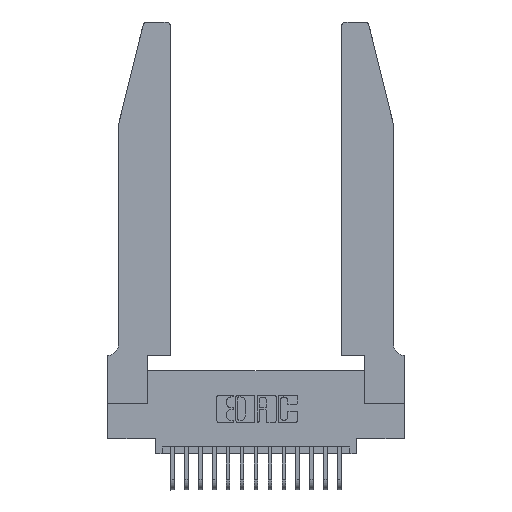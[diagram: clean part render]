
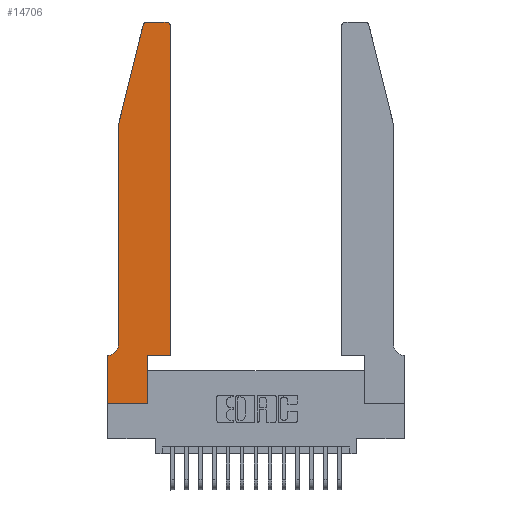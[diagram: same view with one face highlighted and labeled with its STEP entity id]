
A CAD part, top view. The second image highlights one B-rep face of the part: STEP entity #14706.
In plain terms, the highlighted planar face has unit normal (0, 0, 1).
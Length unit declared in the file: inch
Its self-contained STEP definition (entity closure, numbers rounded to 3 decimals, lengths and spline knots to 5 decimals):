
#154 = CIRCLE ( 'NONE', #2143, 0.03 ) ;
#190 = CARTESIAN_POINT ( 'NONE',  ( 0., 0.35, 0.37 ) ) ;
#294 = ORIENTED_EDGE ( 'NONE', *, *, #7424, .T. ) ;
#326 = CARTESIAN_POINT ( 'NONE',  ( 0.0755, 0.42, 0.37 ) ) ;
#828 = LINE ( 'NONE', #13875, #15801 ) ;
#1557 = VERTEX_POINT ( 'NONE', #5590 ) ;
#1702 = ORIENTED_EDGE ( 'NONE', *, *, #6084, .T. ) ;
#1766 = DIRECTION ( 'NONE',  ( 1., 0., 0. ) ) ;
#1769 = LINE ( 'NONE', #11265, #7815 ) ;
#1826 = CARTESIAN_POINT ( 'NONE',  ( 0.2865, 0.35, 0.37 ) ) ;
#1850 = VERTEX_POINT ( 'NONE', #4550 ) ;
#2143 = AXIS2_PLACEMENT_3D ( 'NONE', #6010, #15923, #7480 ) ;
#2507 = FACE_OUTER_BOUND ( 'NONE', #15853, .T. ) ;
#2542 = EDGE_CURVE ( 'NONE', #5289, #15645, #154, .T. ) ;
#2556 = ORIENTED_EDGE ( 'NONE', *, *, #13626, .T. ) ;
#2882 = AXIS2_PLACEMENT_3D ( 'NONE', #8494, #18285, #9923 ) ;
#2989 = LINE ( 'NONE', #3515, #9884 ) ;
#3036 = VERTEX_POINT ( 'NONE', #9968 ) ;
#3207 = PLANE ( 'NONE',  #17523 ) ;
#3515 = CARTESIAN_POINT ( 'NONE',  ( 0.4505, 0.35, 0.37 ) ) ;
#3634 = VERTEX_POINT ( 'NONE', #12335 ) ;
#3712 = EDGE_CURVE ( 'NONE', #3036, #1557, #828, .T. ) ;
#3813 = DIRECTION ( 'NONE',  ( 0., -1., 0. ) ) ;
#4016 = ORIENTED_EDGE ( 'NONE', *, *, #12811, .T. ) ;
#4052 = LINE ( 'NONE', #1826, #17839 ) ;
#4151 = CARTESIAN_POINT ( 'NONE',  ( 0.0055, 0.35, 0.37 ) ) ;
#4157 = ORIENTED_EDGE ( 'NONE', *, *, #9120, .T. ) ;
#4394 = CIRCLE ( 'NONE', #2882, 0.03 ) ;
#4471 = DIRECTION ( 'NONE',  ( -1., 0., 0. ) ) ;
#4533 = CARTESIAN_POINT ( 'NONE',  ( 0.0055, 0.42, 0.37 ) ) ;
#4550 = CARTESIAN_POINT ( 'NONE',  ( 0.4205, 2.75, 0.37 ) ) ;
#5059 = DIRECTION ( 'NONE',  ( 1., 0., 0. ) ) ;
#5289 = VERTEX_POINT ( 'NONE', #13985 ) ;
#5510 = EDGE_CURVE ( 'NONE', #10821, #3036, #15515, .T. ) ;
#5590 = CARTESIAN_POINT ( 'NONE',  ( 0., 0., 0.37 ) ) ;
#5830 = EDGE_CURVE ( 'NONE', #3634, #6228, #6855, .T. ) ;
#5984 = VECTOR ( 'NONE', #13143, 39.37008 ) ;
#6010 = CARTESIAN_POINT ( 'NONE',  ( 0.284, 2.72, 0.37 ) ) ;
#6017 = DIRECTION ( 'NONE',  ( -1., 0., 0. ) ) ;
#6084 = EDGE_CURVE ( 'NONE', #1557, #15093, #17287, .T. ) ;
#6228 = VERTEX_POINT ( 'NONE', #326 ) ;
#6595 = ORIENTED_EDGE ( 'NONE', *, *, #10957, .T. ) ;
#6855 = LINE ( 'NONE', #13909, #14875 ) ;
#7252 = VERTEX_POINT ( 'NONE', #9466 ) ;
#7266 = AXIS2_PLACEMENT_3D ( 'NONE', #4533, #14559, #6017 ) ;
#7424 = EDGE_CURVE ( 'NONE', #16525, #12437, #8203, .T. ) ;
#7480 = DIRECTION ( 'NONE',  ( 1., 0., 0. ) ) ;
#7580 = VECTOR ( 'NONE', #18557, 39.37008 ) ;
#7815 = VECTOR ( 'NONE', #12733, 39.37008 ) ;
#8203 = LINE ( 'NONE', #17210, #15257 ) ;
#8494 = CARTESIAN_POINT ( 'NONE',  ( 0.4205, 2.72, 0.37 ) ) ;
#8720 = CARTESIAN_POINT ( 'NONE',  ( 0.4505, 0.35, 0.37 ) ) ;
#8847 = DIRECTION ( 'NONE',  ( 0., 1., 0. ) ) ;
#9120 = EDGE_CURVE ( 'NONE', #15093, #7252, #4052, .T. ) ;
#9465 = VECTOR ( 'NONE', #4471, 39.37008 ) ;
#9466 = CARTESIAN_POINT ( 'NONE',  ( 0.2865, 0.35, 0.37 ) ) ;
#9628 = CARTESIAN_POINT ( 'NONE',  ( 0.25487, 2.72718, 0.37 ) ) ;
#9884 = VECTOR ( 'NONE', #5059, 39.37008 ) ;
#9907 = LINE ( 'NONE', #14498, #9465 ) ;
#9923 = DIRECTION ( 'NONE',  ( 1., 0., 0. ) ) ;
#9968 = CARTESIAN_POINT ( 'NONE',  ( 0., 0.35, 0.37 ) ) ;
#10329 = ORIENTED_EDGE ( 'NONE', *, *, #3712, .T. ) ;
#10551 = DIRECTION ( 'NONE',  ( 0., 0., 1. ) ) ;
#10821 = VERTEX_POINT ( 'NONE', #4151 ) ;
#10957 = EDGE_CURVE ( 'NONE', #1850, #5289, #9907, .T. ) ;
#11265 = CARTESIAN_POINT ( 'NONE',  ( 0.0755, 2., 0.37 ) ) ;
#11644 = CARTESIAN_POINT ( 'NONE',  ( 0.0755, 0.35, 0.37 ) ) ;
#11752 = CARTESIAN_POINT ( 'NONE',  ( 0., 0., 0.37 ) ) ;
#12335 = CARTESIAN_POINT ( 'NONE',  ( 0.0755, 2., 0.37 ) ) ;
#12437 = VERTEX_POINT ( 'NONE', #16931 ) ;
#12733 = DIRECTION ( 'NONE',  ( -0.239, -0.971, 0. ) ) ;
#12811 = EDGE_CURVE ( 'NONE', #7252, #16525, #2989, .T. ) ;
#13143 = DIRECTION ( 'NONE',  ( 1., 0., 0. ) ) ;
#13166 = CIRCLE ( 'NONE', #7266, 0.07 ) ;
#13374 = ORIENTED_EDGE ( 'NONE', *, *, #17242, .T. ) ;
#13396 = ORIENTED_EDGE ( 'NONE', *, *, #5510, .T. ) ;
#13626 = EDGE_CURVE ( 'NONE', #12437, #1850, #4394, .T. ) ;
#13875 = CARTESIAN_POINT ( 'NONE',  ( 0., 0., 0.37 ) ) ;
#13909 = CARTESIAN_POINT ( 'NONE',  ( 0.0755, 2., 0.37 ) ) ;
#13924 = ORIENTED_EDGE ( 'NONE', *, *, #15940, .T. ) ;
#13985 = CARTESIAN_POINT ( 'NONE',  ( 0.284, 2.75, 0.37 ) ) ;
#14480 = CARTESIAN_POINT ( 'NONE',  ( 0.2865, 0., 0.37 ) ) ;
#14498 = CARTESIAN_POINT ( 'NONE',  ( 0.2605, 2.75, 0.37 ) ) ;
#14559 = DIRECTION ( 'NONE',  ( 0., 0., -1. ) ) ;
#14706 = ADVANCED_FACE ( 'NONE', ( #2507 ), #3207, .T. ) ;
#14875 = VECTOR ( 'NONE', #3813, 39.37008 ) ;
#15093 = VERTEX_POINT ( 'NONE', #14480 ) ;
#15254 = DIRECTION ( 'NONE',  ( 0., -1., 0. ) ) ;
#15257 = VECTOR ( 'NONE', #8847, 39.37008 ) ;
#15515 = LINE ( 'NONE', #11644, #7580 ) ;
#15645 = VERTEX_POINT ( 'NONE', #9628 ) ;
#15801 = VECTOR ( 'NONE', #15254, 39.37008 ) ;
#15853 = EDGE_LOOP ( 'NONE', ( #6595, #18509, #13374, #17675, #13924, #13396, #10329, #1702, #4157, #4016, #294, #2556 ) ) ;
#15923 = DIRECTION ( 'NONE',  ( 0., 0., 1. ) ) ;
#15940 = EDGE_CURVE ( 'NONE', #6228, #10821, #13166, .T. ) ;
#16234 = DIRECTION ( 'NONE',  ( 0., 1., 0. ) ) ;
#16525 = VERTEX_POINT ( 'NONE', #8720 ) ;
#16931 = CARTESIAN_POINT ( 'NONE',  ( 0.4505, 2.72, 0.37 ) ) ;
#17210 = CARTESIAN_POINT ( 'NONE',  ( 0.4505, 0.35, 0.37 ) ) ;
#17242 = EDGE_CURVE ( 'NONE', #15645, #3634, #1769, .T. ) ;
#17287 = LINE ( 'NONE', #11752, #5984 ) ;
#17523 = AXIS2_PLACEMENT_3D ( 'NONE', #190, #10551, #1766 ) ;
#17675 = ORIENTED_EDGE ( 'NONE', *, *, #5830, .T. ) ;
#17839 = VECTOR ( 'NONE', #16234, 39.37008 ) ;
#18285 = DIRECTION ( 'NONE',  ( 0., 0., 1. ) ) ;
#18509 = ORIENTED_EDGE ( 'NONE', *, *, #2542, .T. ) ;
#18557 = DIRECTION ( 'NONE',  ( -1., 0., 0. ) ) ;
